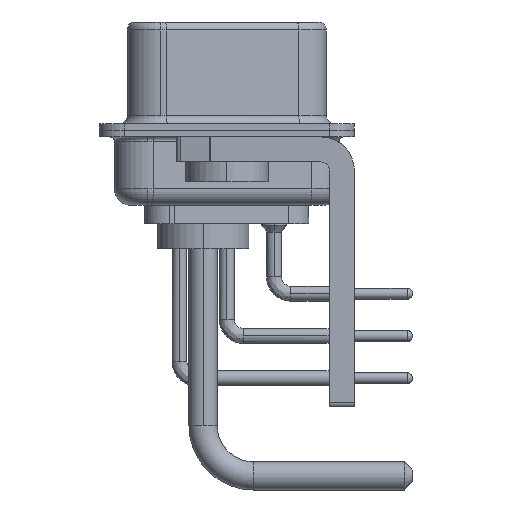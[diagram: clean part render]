
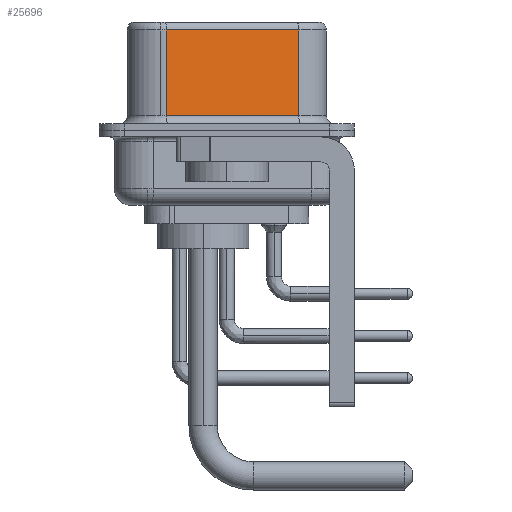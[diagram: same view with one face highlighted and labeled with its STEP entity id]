
A CAD part, left-side view. The second image highlights one B-rep face of the part: STEP entity #25696.
In plain terms, the highlighted planar face has unit normal (-0.985, -0.174, 0).
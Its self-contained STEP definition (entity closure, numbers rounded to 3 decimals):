
#1113 = CARTESIAN_POINT ( 'NONE',  ( 3.73, 3.628, 6.52 ) ) ;
#1511 = VERTEX_POINT ( 'NONE', #29151 ) ;
#1861 = ORIENTED_EDGE ( 'NONE', *, *, #33645, .T. ) ;
#2295 = DIRECTION ( 'NONE',  ( 0., 0., -1. ) ) ;
#4091 = ORIENTED_EDGE ( 'NONE', *, *, #19475, .F. ) ;
#4116 = DIRECTION ( 'NONE',  ( -0.174, 0.985, 0. ) ) ;
#4466 = DIRECTION ( 'NONE',  ( 0.985, 0.174, 0. ) ) ;
#4741 = AXIS2_PLACEMENT_3D ( 'NONE', #31882, #4466, #4116 ) ;
#5363 = ORIENTED_EDGE ( 'NONE', *, *, #10903, .T. ) ;
#6166 = CARTESIAN_POINT ( 'NONE',  ( 5.132, -4.322, 6.02 ) ) ;
#10140 = CARTESIAN_POINT ( 'NONE',  ( 5.132, -4.322, 0.9 ) ) ;
#10290 = VERTEX_POINT ( 'NONE', #6166 ) ;
#10489 = LINE ( 'NONE', #10140, #29087 ) ;
#10903 = EDGE_CURVE ( 'NONE', #10290, #29975, #34558, .T. ) ;
#12154 = LINE ( 'NONE', #1113, #23727 ) ;
#12164 = CARTESIAN_POINT ( 'NONE',  ( 5.132, -4.322, 6.02 ) ) ;
#14129 = EDGE_CURVE ( 'NONE', #29975, #25273, #12154, .T. ) ;
#14515 = VECTOR ( 'NONE', #31906, 1000. ) ;
#15782 = CARTESIAN_POINT ( 'NONE',  ( 3.73, 3.628, 0.9 ) ) ;
#17674 = FACE_OUTER_BOUND ( 'NONE', #27535, .T. ) ;
#18668 = LINE ( 'NONE', #24169, #18725 ) ;
#18725 = VECTOR ( 'NONE', #35170, 1000. ) ;
#19475 = EDGE_CURVE ( 'NONE', #10290, #1511, #18668, .T. ) ;
#21053 = PLANE ( 'NONE',  #4741 ) ;
#23727 = VECTOR ( 'NONE', #2295, 1000. ) ;
#24169 = CARTESIAN_POINT ( 'NONE',  ( 5.132, -4.322, 6.52 ) ) ;
#25273 = VERTEX_POINT ( 'NONE', #15782 ) ;
#25696 = ADVANCED_FACE ( 'NONE', ( #17674 ), #21053, .F. ) ;
#25802 = CARTESIAN_POINT ( 'NONE',  ( 3.73, 3.628, 6.02 ) ) ;
#27535 = EDGE_LOOP ( 'NONE', ( #4091, #5363, #34031, #1861 ) ) ;
#29087 = VECTOR ( 'NONE', #31851, 1000. ) ;
#29151 = CARTESIAN_POINT ( 'NONE',  ( 5.132, -4.322, 0.9 ) ) ;
#29975 = VERTEX_POINT ( 'NONE', #25802 ) ;
#31851 = DIRECTION ( 'NONE',  ( 0.174, -0.985, 0. ) ) ;
#31882 = CARTESIAN_POINT ( 'NONE',  ( 5.132, -4.322, 6.52 ) ) ;
#31906 = DIRECTION ( 'NONE',  ( -0.174, 0.985, 0. ) ) ;
#33645 = EDGE_CURVE ( 'NONE', #25273, #1511, #10489, .T. ) ;
#34031 = ORIENTED_EDGE ( 'NONE', *, *, #14129, .T. ) ;
#34558 = LINE ( 'NONE', #12164, #14515 ) ;
#35170 = DIRECTION ( 'NONE',  ( 0., 0., -1. ) ) ;
